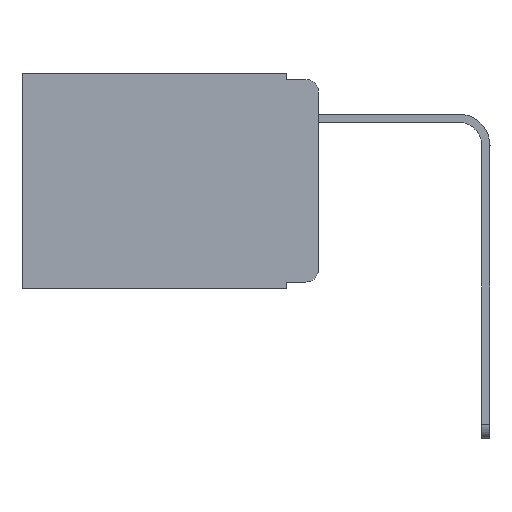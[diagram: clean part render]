
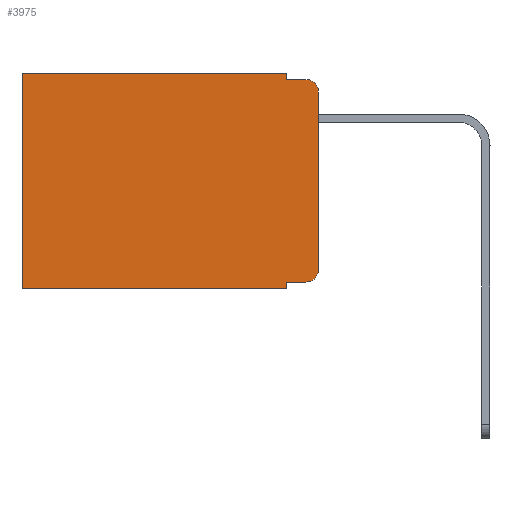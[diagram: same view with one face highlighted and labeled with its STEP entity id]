
A CAD part, left-side view. The second image highlights one B-rep face of the part: STEP entity #3975.
In plain terms, the highlighted planar face has unit normal (-1, 0, 0).
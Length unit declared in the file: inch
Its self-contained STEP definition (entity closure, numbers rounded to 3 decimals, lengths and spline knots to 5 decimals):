
#272 = DIRECTION ( 'NONE',  ( 0., 0., -1. ) ) ;
#276 = LINE ( 'NONE', #20242, #12811 ) ;
#577 = LINE ( 'NONE', #11723, #13621 ) ;
#812 = LINE ( 'NONE', #5835, #17101 ) ;
#866 = AXIS2_PLACEMENT_3D ( 'NONE', #15738, #18984, #6400 ) ;
#1013 = CARTESIAN_POINT ( 'NONE',  ( 0.298, 0.051, 0. ) ) ;
#1246 = VECTOR ( 'NONE', #16281, 39.37008 ) ;
#2003 = ORIENTED_EDGE ( 'NONE', *, *, #7058, .T. ) ;
#2039 = EDGE_CURVE ( 'NONE', #20161, #4234, #15580, .T. ) ;
#2126 = DIRECTION ( 'NONE',  ( 0., -1., 0. ) ) ;
#2206 = ORIENTED_EDGE ( 'NONE', *, *, #13554, .T. ) ;
#2209 = EDGE_CURVE ( 'NONE', #12212, #14226, #276, .T. ) ;
#2783 = ORIENTED_EDGE ( 'NONE', *, *, #2039, .F. ) ;
#2877 = ORIENTED_EDGE ( 'NONE', *, *, #10889, .F. ) ;
#3084 = CARTESIAN_POINT ( 'NONE',  ( 0.298, 0., -0.343 ) ) ;
#3087 = CARTESIAN_POINT ( 'NONE',  ( 0.298, 0.02, -0.313 ) ) ;
#3148 = CIRCLE ( 'NONE', #16406, 0.02 ) ;
#3269 = CARTESIAN_POINT ( 'NONE',  ( 0.298, 0.02, -0.03 ) ) ;
#3645 = CARTESIAN_POINT ( 'NONE',  ( 0.298, 0.051, -0.01 ) ) ;
#3739 = CARTESIAN_POINT ( 'NONE',  ( 0.298, 0.473, -0.343 ) ) ;
#3975 = ADVANCED_FACE ( 'NONE', ( #12019 ), #18850, .F. ) ;
#4077 = VERTEX_POINT ( 'NONE', #12102 ) ;
#4234 = VERTEX_POINT ( 'NONE', #15102 ) ;
#4482 = CARTESIAN_POINT ( 'NONE',  ( 0.298, 0.051, 0. ) ) ;
#4609 = CARTESIAN_POINT ( 'NONE',  ( 0.298, 0.02, -0.333 ) ) ;
#4864 = ORIENTED_EDGE ( 'NONE', *, *, #2209, .F. ) ;
#5450 = DIRECTION ( 'NONE',  ( 0., 0., -1. ) ) ;
#5755 = CARTESIAN_POINT ( 'NONE',  ( 0.298, 0.473, 0. ) ) ;
#5818 = DIRECTION ( 'NONE',  ( 0., 0., -1. ) ) ;
#5835 = CARTESIAN_POINT ( 'NONE',  ( 0.298, 0., 0. ) ) ;
#5952 = CARTESIAN_POINT ( 'NONE',  ( 0.298, 0.051, -0.333 ) ) ;
#6008 = LINE ( 'NONE', #14653, #18622 ) ;
#6073 = EDGE_CURVE ( 'NONE', #12740, #6085, #6008, .T. ) ;
#6085 = VERTEX_POINT ( 'NONE', #3739 ) ;
#6090 = DIRECTION ( 'NONE',  ( 0., 0., -1. ) ) ;
#6400 = DIRECTION ( 'NONE',  ( 0., 0., -1. ) ) ;
#6708 = EDGE_CURVE ( 'NONE', #11700, #12924, #577, .T. ) ;
#6926 = LINE ( 'NONE', #8427, #12575 ) ;
#7058 = EDGE_CURVE ( 'NONE', #11700, #12740, #812, .T. ) ;
#7341 = ORIENTED_EDGE ( 'NONE', *, *, #17168, .T. ) ;
#7916 = AXIS2_PLACEMENT_3D ( 'NONE', #3087, #15864, #14329 ) ;
#8417 = LINE ( 'NONE', #3645, #1246 ) ;
#8427 = CARTESIAN_POINT ( 'NONE',  ( 0.298, 0.051, -0.333 ) ) ;
#8497 = CARTESIAN_POINT ( 'NONE',  ( 0.298, 0.051, -0.01 ) ) ;
#8519 = DIRECTION ( 'NONE',  ( 0., 0., -1. ) ) ;
#8522 = EDGE_CURVE ( 'NONE', #20161, #14363, #6926, .T. ) ;
#8599 = EDGE_CURVE ( 'NONE', #12924, #4077, #8417, .T. ) ;
#10889 = EDGE_CURVE ( 'NONE', #4234, #6085, #16207, .T. ) ;
#11076 = DIRECTION ( 'NONE',  ( 0., 1., 0. ) ) ;
#11700 = VERTEX_POINT ( 'NONE', #4482 ) ;
#11723 = CARTESIAN_POINT ( 'NONE',  ( 0.298, 0.051, 0. ) ) ;
#12019 = FACE_OUTER_BOUND ( 'NONE', #17958, .T. ) ;
#12102 = CARTESIAN_POINT ( 'NONE',  ( 0.298, 0.02, -0.01 ) ) ;
#12212 = VERTEX_POINT ( 'NONE', #16820 ) ;
#12400 = ORIENTED_EDGE ( 'NONE', *, *, #6073, .T. ) ;
#12575 = VECTOR ( 'NONE', #2126, 39.37008 ) ;
#12740 = VERTEX_POINT ( 'NONE', #5755 ) ;
#12811 = VECTOR ( 'NONE', #6090, 39.37008 ) ;
#12821 = ORIENTED_EDGE ( 'NONE', *, *, #8599, .F. ) ;
#12924 = VERTEX_POINT ( 'NONE', #8497 ) ;
#13554 = EDGE_CURVE ( 'NONE', #14363, #14226, #20096, .T. ) ;
#13621 = VECTOR ( 'NONE', #5450, 39.37008 ) ;
#13712 = VECTOR ( 'NONE', #11076, 39.37008 ) ;
#14226 = VERTEX_POINT ( 'NONE', #15635 ) ;
#14329 = DIRECTION ( 'NONE',  ( 0., 0., -1. ) ) ;
#14363 = VERTEX_POINT ( 'NONE', #4609 ) ;
#14653 = CARTESIAN_POINT ( 'NONE',  ( 0.298, 0.473, 0. ) ) ;
#15072 = VECTOR ( 'NONE', #5818, 39.37008 ) ;
#15102 = CARTESIAN_POINT ( 'NONE',  ( 0.298, 0.051, -0.343 ) ) ;
#15580 = LINE ( 'NONE', #1013, #15072 ) ;
#15635 = CARTESIAN_POINT ( 'NONE',  ( 0.298, 0., -0.313 ) ) ;
#15738 = CARTESIAN_POINT ( 'NONE',  ( 0.298, 0., 0. ) ) ;
#15864 = DIRECTION ( 'NONE',  ( -1., 0., 0. ) ) ;
#16207 = LINE ( 'NONE', #3084, #13712 ) ;
#16281 = DIRECTION ( 'NONE',  ( 0., -1., 0. ) ) ;
#16406 = AXIS2_PLACEMENT_3D ( 'NONE', #3269, #19032, #272 ) ;
#16464 = ORIENTED_EDGE ( 'NONE', *, *, #6708, .F. ) ;
#16820 = CARTESIAN_POINT ( 'NONE',  ( 0.298, 0., -0.03 ) ) ;
#17101 = VECTOR ( 'NONE', #19864, 39.37008 ) ;
#17168 = EDGE_CURVE ( 'NONE', #12212, #4077, #3148, .T. ) ;
#17958 = EDGE_LOOP ( 'NONE', ( #4864, #7341, #12821, #16464, #2003, #12400, #2877, #2783, #19440, #2206 ) ) ;
#18622 = VECTOR ( 'NONE', #8519, 39.37008 ) ;
#18850 = PLANE ( 'NONE',  #866 ) ;
#18984 = DIRECTION ( 'NONE',  ( 1., 0., 0. ) ) ;
#19032 = DIRECTION ( 'NONE',  ( -1., 0., 0. ) ) ;
#19440 = ORIENTED_EDGE ( 'NONE', *, *, #8522, .T. ) ;
#19864 = DIRECTION ( 'NONE',  ( 0., 1., 0. ) ) ;
#20096 = CIRCLE ( 'NONE', #7916, 0.02 ) ;
#20161 = VERTEX_POINT ( 'NONE', #5952 ) ;
#20242 = CARTESIAN_POINT ( 'NONE',  ( 0.298, 0., 0. ) ) ;
